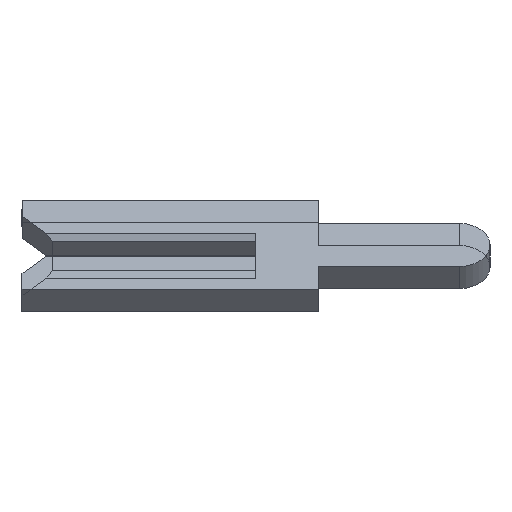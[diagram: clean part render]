
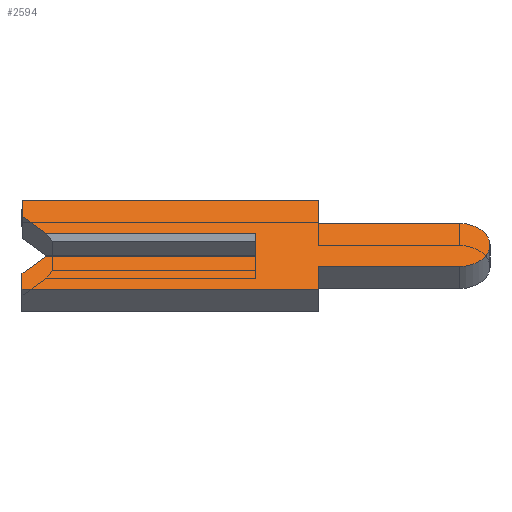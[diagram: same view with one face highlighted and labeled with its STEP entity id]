
A CAD part, left-side view. The second image highlights one B-rep face of the part: STEP entity #2594.
In plain terms, the highlighted face is planar.
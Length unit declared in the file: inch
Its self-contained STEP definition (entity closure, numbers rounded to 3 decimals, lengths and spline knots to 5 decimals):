
#57 = LINE ( 'NONE', #77, #2886 ) ;
#64 = LINE ( 'NONE', #4101, #4122 ) ;
#77 = CARTESIAN_POINT ( 'NONE',  ( -0.01, 0.15, 0.026 ) ) ;
#119 = ORIENTED_EDGE ( 'NONE', *, *, #3250, .F. ) ;
#123 = DIRECTION ( 'NONE',  ( 1., 0., 0. ) ) ;
#203 = ORIENTED_EDGE ( 'NONE', *, *, #1824, .F. ) ;
#213 = VERTEX_POINT ( 'NONE', #3388 ) ;
#237 = ORIENTED_EDGE ( 'NONE', *, *, #956, .F. ) ;
#280 = ORIENTED_EDGE ( 'NONE', *, *, #2459, .F. ) ;
#323 = VECTOR ( 'NONE', #3633, 39.37008 ) ;
#337 = CARTESIAN_POINT ( 'NONE',  ( -0.01, -0.04, -0.04 ) ) ;
#389 = ORIENTED_EDGE ( 'NONE', *, *, #1911, .F. ) ;
#533 = ORIENTED_EDGE ( 'NONE', *, *, #2974, .F. ) ;
#574 = CARTESIAN_POINT ( 'NONE',  ( -0.01, -0.1305, 0.0195 ) ) ;
#582 = EDGE_CURVE ( 'NONE', #213, #1079, #64, .T. ) ;
#589 = LINE ( 'NONE', #4257, #967 ) ;
#680 = DIRECTION ( 'NONE',  ( 0., -1., 0. ) ) ;
#795 = DIRECTION ( 'NONE',  ( 0., 0., -1. ) ) ;
#837 = VERTEX_POINT ( 'NONE', #1029 ) ;
#839 = PLANE ( 'NONE',  #3557 ) ;
#867 = VERTEX_POINT ( 'NONE', #337 ) ;
#868 = EDGE_CURVE ( 'NONE', #3542, #2663, #1648, .T. ) ;
#924 = EDGE_CURVE ( 'NONE', #1150, #837, #970, .T. ) ;
#956 = EDGE_CURVE ( 'NONE', #867, #1036, #3637, .T. ) ;
#967 = VECTOR ( 'NONE', #3947, 39.37008 ) ;
#970 = LINE ( 'NONE', #3431, #1490 ) ;
#1011 = CARTESIAN_POINT ( 'NONE',  ( -0.01, -0.1305, -0.01 ) ) ;
#1029 = CARTESIAN_POINT ( 'NONE',  ( -0.01, 0.15, 0.026 ) ) ;
#1036 = VERTEX_POINT ( 'NONE', #3155 ) ;
#1063 = CARTESIAN_POINT ( 'NONE',  ( -0.01, 0.15, -0.04 ) ) ;
#1076 = CARTESIAN_POINT ( 'NONE',  ( -0.01, -0.1305, 0. ) ) ;
#1079 = VERTEX_POINT ( 'NONE', #2757 ) ;
#1084 = CIRCLE ( 'NONE', #3354, 0.0195 ) ;
#1134 = VERTEX_POINT ( 'NONE', #1416 ) ;
#1147 = EDGE_CURVE ( 'NONE', #2663, #2560, #2244, .T. ) ;
#1150 = VERTEX_POINT ( 'NONE', #3449 ) ;
#1171 = CARTESIAN_POINT ( 'NONE',  ( -0.01, 0., -0.01 ) ) ;
#1176 = VERTEX_POINT ( 'NONE', #2049 ) ;
#1194 = ORIENTED_EDGE ( 'NONE', *, *, #868, .F. ) ;
#1314 = VECTOR ( 'NONE', #4107, 39.37008 ) ;
#1416 = CARTESIAN_POINT ( 'NONE',  ( -0.01, -0.04, -0.0195 ) ) ;
#1490 = VECTOR ( 'NONE', #3138, 39.37008 ) ;
#1550 = CARTESIAN_POINT ( 'NONE',  ( -0.01, 0.15, 0.01 ) ) ;
#1562 = CARTESIAN_POINT ( 'NONE',  ( -0.01, -0.04, 0.04 ) ) ;
#1645 = VECTOR ( 'NONE', #795, 39.37008 ) ;
#1648 = LINE ( 'NONE', #1011, #1762 ) ;
#1753 = EDGE_LOOP ( 'NONE', ( #3398, #2996, #1194, #3053, #1917, #237, #533, #389, #203, #280, #119, #3606, #4336, #4151 ) ) ;
#1754 = LINE ( 'NONE', #3608, #2783 ) ;
#1762 = VECTOR ( 'NONE', #680, 39.37008 ) ;
#1824 = EDGE_CURVE ( 'NONE', #3846, #2198, #1084, .T. ) ;
#1855 = CARTESIAN_POINT ( 'NONE',  ( -0.01, -0.1305, 0. ) ) ;
#1868 = VECTOR ( 'NONE', #2130, 39.37008 ) ;
#1911 = EDGE_CURVE ( 'NONE', #2198, #1134, #2724, .T. ) ;
#1917 = ORIENTED_EDGE ( 'NONE', *, *, #3973, .F. ) ;
#1985 = CARTESIAN_POINT ( 'NONE',  ( -0.01, 0.15, -0.026 ) ) ;
#2049 = CARTESIAN_POINT ( 'NONE',  ( -0.01, 0.15, -0.026 ) ) ;
#2079 = VERTEX_POINT ( 'NONE', #3879 ) ;
#2086 = VECTOR ( 'NONE', #2544, 39.37008 ) ;
#2130 = DIRECTION ( 'NONE',  ( 0., 1., 0. ) ) ;
#2152 = EDGE_CURVE ( 'NONE', #837, #213, #57, .T. ) ;
#2198 = VERTEX_POINT ( 'NONE', #4244 ) ;
#2217 = DIRECTION ( 'NONE',  ( 0., 0., -1. ) ) ;
#2244 = LINE ( 'NONE', #2456, #1314 ) ;
#2347 = VECTOR ( 'NONE', #4119, 39.37008 ) ;
#2456 = CARTESIAN_POINT ( 'NONE',  ( -0.01, 0., 0.0065 ) ) ;
#2459 = EDGE_CURVE ( 'NONE', #2079, #3846, #1754, .T. ) ;
#2544 = DIRECTION ( 'NONE',  ( 0., -1., 0. ) ) ;
#2560 = VERTEX_POINT ( 'NONE', #2586 ) ;
#2561 = DIRECTION ( 'NONE',  ( 0., -1., 0. ) ) ;
#2586 = CARTESIAN_POINT ( 'NONE',  ( -0.01, 0., 0.01 ) ) ;
#2594 = ADVANCED_FACE ( 'NONE', ( #3632 ), #839, .F. ) ;
#2630 = DIRECTION ( 'NONE',  ( 0., 0., 1. ) ) ;
#2663 = VERTEX_POINT ( 'NONE', #1171 ) ;
#2687 = EDGE_CURVE ( 'NONE', #1150, #2560, #3683, .T. ) ;
#2724 = LINE ( 'NONE', #3835, #1868 ) ;
#2757 = CARTESIAN_POINT ( 'NONE',  ( -0.01, -0.04, 0.04 ) ) ;
#2783 = VECTOR ( 'NONE', #2561, 39.37008 ) ;
#2815 = DIRECTION ( 'NONE',  ( 0., 0., 1. ) ) ;
#2886 = VECTOR ( 'NONE', #2815, 39.37008 ) ;
#2974 = EDGE_CURVE ( 'NONE', #1134, #867, #589, .T. ) ;
#2996 = ORIENTED_EDGE ( 'NONE', *, *, #1147, .F. ) ;
#3018 = CARTESIAN_POINT ( 'NONE',  ( -0.01, 0.1305, -0.0065 ) ) ;
#3053 = ORIENTED_EDGE ( 'NONE', *, *, #4298, .F. ) ;
#3138 = DIRECTION ( 'NONE',  ( 0., 0.707, 0.707 ) ) ;
#3155 = CARTESIAN_POINT ( 'NONE',  ( -0.01, 0.15, -0.04 ) ) ;
#3198 = DIRECTION ( 'NONE',  ( 0., 0., -1. ) ) ;
#3214 = LINE ( 'NONE', #3018, #323 ) ;
#3250 = EDGE_CURVE ( 'NONE', #1079, #2079, #3483, .T. ) ;
#3354 = AXIS2_PLACEMENT_3D ( 'NONE', #1076, #3867, #3198 ) ;
#3388 = CARTESIAN_POINT ( 'NONE',  ( -0.01, 0.15, 0.04 ) ) ;
#3398 = ORIENTED_EDGE ( 'NONE', *, *, #2687, .T. ) ;
#3404 = DIRECTION ( 'NONE',  ( 0., -1., 0. ) ) ;
#3431 = CARTESIAN_POINT ( 'NONE',  ( -0.01, 0.1305, 0.0065 ) ) ;
#3449 = CARTESIAN_POINT ( 'NONE',  ( -0.01, 0.134, 0.01 ) ) ;
#3483 = LINE ( 'NONE', #1562, #1645 ) ;
#3542 = VERTEX_POINT ( 'NONE', #4337 ) ;
#3557 = AXIS2_PLACEMENT_3D ( 'NONE', #1855, #123, #2217 ) ;
#3606 = ORIENTED_EDGE ( 'NONE', *, *, #582, .F. ) ;
#3608 = CARTESIAN_POINT ( 'NONE',  ( -0.01, -0.04, 0.0195 ) ) ;
#3632 = FACE_OUTER_BOUND ( 'NONE', #1753, .T. ) ;
#3633 = DIRECTION ( 'NONE',  ( 0., -0.707, 0.707 ) ) ;
#3637 = LINE ( 'NONE', #1063, #2347 ) ;
#3683 = LINE ( 'NONE', #1550, #2086 ) ;
#3736 = VECTOR ( 'NONE', #2630, 39.37008 ) ;
#3835 = CARTESIAN_POINT ( 'NONE',  ( -0.01, -0.04, -0.0195 ) ) ;
#3846 = VERTEX_POINT ( 'NONE', #574 ) ;
#3867 = DIRECTION ( 'NONE',  ( 1., 0., 0. ) ) ;
#3879 = CARTESIAN_POINT ( 'NONE',  ( -0.01, -0.04, 0.0195 ) ) ;
#3947 = DIRECTION ( 'NONE',  ( 0., 0., -1. ) ) ;
#3973 = EDGE_CURVE ( 'NONE', #1036, #1176, #4064, .T. ) ;
#4064 = LINE ( 'NONE', #1985, #3736 ) ;
#4101 = CARTESIAN_POINT ( 'NONE',  ( -0.01, 0.15, 0.04 ) ) ;
#4107 = DIRECTION ( 'NONE',  ( 0., 0., 1. ) ) ;
#4119 = DIRECTION ( 'NONE',  ( 0., 1., 0. ) ) ;
#4122 = VECTOR ( 'NONE', #3404, 39.37008 ) ;
#4151 = ORIENTED_EDGE ( 'NONE', *, *, #924, .F. ) ;
#4244 = CARTESIAN_POINT ( 'NONE',  ( -0.01, -0.1305, -0.0195 ) ) ;
#4257 = CARTESIAN_POINT ( 'NONE',  ( -0.01, -0.04, -0.04 ) ) ;
#4298 = EDGE_CURVE ( 'NONE', #1176, #3542, #3214, .T. ) ;
#4336 = ORIENTED_EDGE ( 'NONE', *, *, #2152, .F. ) ;
#4337 = CARTESIAN_POINT ( 'NONE',  ( -0.01, 0.134, -0.01 ) ) ;
